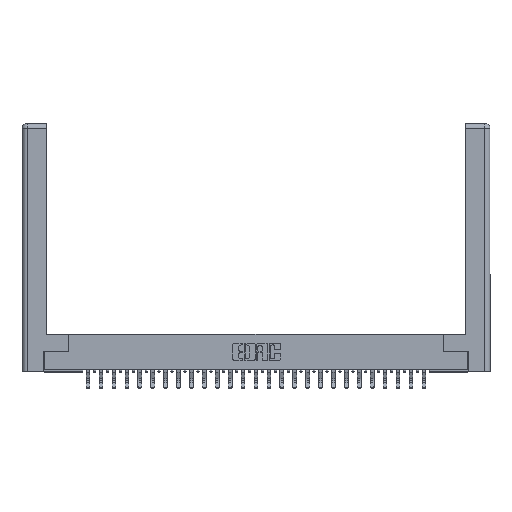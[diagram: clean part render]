
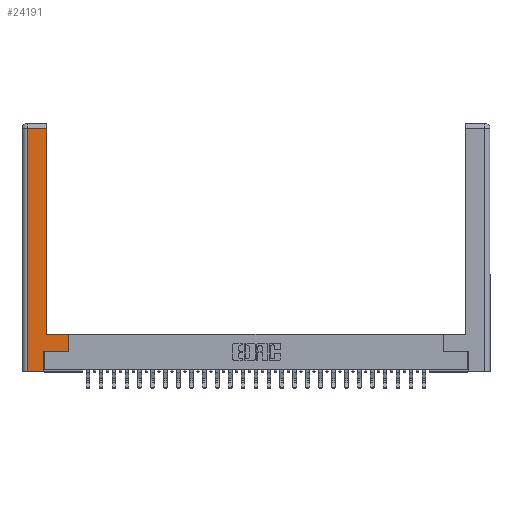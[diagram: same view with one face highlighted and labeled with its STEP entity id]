
A CAD part, top view. The second image highlights one B-rep face of the part: STEP entity #24191.
In plain terms, the highlighted planar face has unit normal (0, 0, 1).
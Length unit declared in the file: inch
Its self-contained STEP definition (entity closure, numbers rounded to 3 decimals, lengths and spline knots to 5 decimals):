
#331 = CARTESIAN_POINT ( 'NONE',  ( 0.295, 0.45, 0. ) ) ;
#437 = CARTESIAN_POINT ( 'NONE',  ( 0.0615, 0., 0. ) ) ;
#684 = EDGE_CURVE ( 'NONE', #1767, #5368, #4535, .T. ) ;
#1240 = EDGE_CURVE ( 'NONE', #6321, #13951, #22969, .T. ) ;
#1262 = DIRECTION ( 'NONE',  ( -1., 0., 0. ) ) ;
#1518 = ORIENTED_EDGE ( 'NONE', *, *, #684, .T. ) ;
#1753 = CARTESIAN_POINT ( 'NONE',  ( 0.0615, 0., 0. ) ) ;
#1767 = VERTEX_POINT ( 'NONE', #18378 ) ;
#1862 = VERTEX_POINT ( 'NONE', #331 ) ;
#2453 = EDGE_LOOP ( 'NONE', ( #29309, #1518, #18646, #12718, #12128, #3135, #28327, #9006 ) ) ;
#2523 = VECTOR ( 'NONE', #1262, 39.37008 ) ;
#3135 = ORIENTED_EDGE ( 'NONE', *, *, #4455, .T. ) ;
#3917 = EDGE_CURVE ( 'NONE', #5368, #19155, #8905, .T. ) ;
#4455 = EDGE_CURVE ( 'NONE', #13951, #30497, #22371, .T. ) ;
#4535 = LINE ( 'NONE', #12998, #30350 ) ;
#4782 = VECTOR ( 'NONE', #27043, 39.37008 ) ;
#5368 = VERTEX_POINT ( 'NONE', #5792 ) ;
#5792 = CARTESIAN_POINT ( 'NONE',  ( 0.0615, 2.94, 0. ) ) ;
#6321 = VERTEX_POINT ( 'NONE', #12071 ) ;
#6531 = CARTESIAN_POINT ( 'NONE',  ( 0.565, 0.245, 0. ) ) ;
#6582 = CARTESIAN_POINT ( 'NONE',  ( 0.295, 0.45, 0. ) ) ;
#6643 = CARTESIAN_POINT ( 'NONE',  ( 0.295, 3., 0. ) ) ;
#7283 = EDGE_CURVE ( 'NONE', #30497, #9797, #30414, .T. ) ;
#8254 = EDGE_CURVE ( 'NONE', #19155, #6321, #9070, .T. ) ;
#8793 = DIRECTION ( 'NONE',  ( 0., 1., 0. ) ) ;
#8905 = LINE ( 'NONE', #437, #4782 ) ;
#9006 = ORIENTED_EDGE ( 'NONE', *, *, #24687, .T. ) ;
#9044 = DIRECTION ( 'NONE',  ( 0., 1., 0. ) ) ;
#9070 = LINE ( 'NONE', #15798, #28706 ) ;
#9513 = LINE ( 'NONE', #6582, #2523 ) ;
#9797 = VERTEX_POINT ( 'NONE', #16308 ) ;
#12071 = CARTESIAN_POINT ( 'NONE',  ( 0.265, 0., 0. ) ) ;
#12128 = ORIENTED_EDGE ( 'NONE', *, *, #1240, .T. ) ;
#12567 = CARTESIAN_POINT ( 'NONE',  ( 0.565, 0.45, 0. ) ) ;
#12718 = ORIENTED_EDGE ( 'NONE', *, *, #8254, .T. ) ;
#12734 = DIRECTION ( 'NONE',  ( 1., 0., 0. ) ) ;
#12998 = CARTESIAN_POINT ( 'NONE',  ( 0.0615, 2.94, 0. ) ) ;
#13951 = VERTEX_POINT ( 'NONE', #21506 ) ;
#15696 = VECTOR ( 'NONE', #9044, 39.37008 ) ;
#15798 = CARTESIAN_POINT ( 'NONE',  ( 0.265, 0., 0. ) ) ;
#16308 = CARTESIAN_POINT ( 'NONE',  ( 0.565, 0.45, 0. ) ) ;
#18378 = CARTESIAN_POINT ( 'NONE',  ( 0.295, 2.94, 0. ) ) ;
#18646 = ORIENTED_EDGE ( 'NONE', *, *, #3917, .T. ) ;
#18654 = PLANE ( 'NONE',  #33611 ) ;
#18982 = DIRECTION ( 'NONE',  ( -1., 0., 0. ) ) ;
#19155 = VERTEX_POINT ( 'NONE', #1753 ) ;
#19468 = DIRECTION ( 'NONE',  ( 1., 0., 0. ) ) ;
#19802 = FACE_OUTER_BOUND ( 'NONE', #2453, .T. ) ;
#20224 = LINE ( 'NONE', #6643, #15696 ) ;
#21506 = CARTESIAN_POINT ( 'NONE',  ( 0.265, 0.245, 0. ) ) ;
#22371 = LINE ( 'NONE', #6531, #29328 ) ;
#22969 = LINE ( 'NONE', #24490, #30754 ) ;
#23635 = DIRECTION ( 'NONE',  ( -1., 0., 0. ) ) ;
#24191 = ADVANCED_FACE ( 'NONE', ( #19802 ), #18654, .F. ) ;
#24490 = CARTESIAN_POINT ( 'NONE',  ( 0.265, 0.245, 0. ) ) ;
#24687 = EDGE_CURVE ( 'NONE', #9797, #1862, #9513, .T. ) ;
#25820 = DIRECTION ( 'NONE',  ( 0., 1., 0. ) ) ;
#27043 = DIRECTION ( 'NONE',  ( 0., -1., 0. ) ) ;
#28327 = ORIENTED_EDGE ( 'NONE', *, *, #7283, .T. ) ;
#28706 = VECTOR ( 'NONE', #12734, 39.37008 ) ;
#29161 = CARTESIAN_POINT ( 'NONE',  ( 0., 0., 0. ) ) ;
#29309 = ORIENTED_EDGE ( 'NONE', *, *, #31890, .T. ) ;
#29328 = VECTOR ( 'NONE', #19468, 39.37008 ) ;
#29404 = DIRECTION ( 'NONE',  ( 0., 0., -1. ) ) ;
#30350 = VECTOR ( 'NONE', #23635, 39.37008 ) ;
#30414 = LINE ( 'NONE', #12567, #32015 ) ;
#30497 = VERTEX_POINT ( 'NONE', #33384 ) ;
#30754 = VECTOR ( 'NONE', #8793, 39.37008 ) ;
#31890 = EDGE_CURVE ( 'NONE', #1862, #1767, #20224, .T. ) ;
#32015 = VECTOR ( 'NONE', #25820, 39.37008 ) ;
#33384 = CARTESIAN_POINT ( 'NONE',  ( 0.565, 0.245, 0. ) ) ;
#33611 = AXIS2_PLACEMENT_3D ( 'NONE', #29161, #29404, #18982 ) ;
